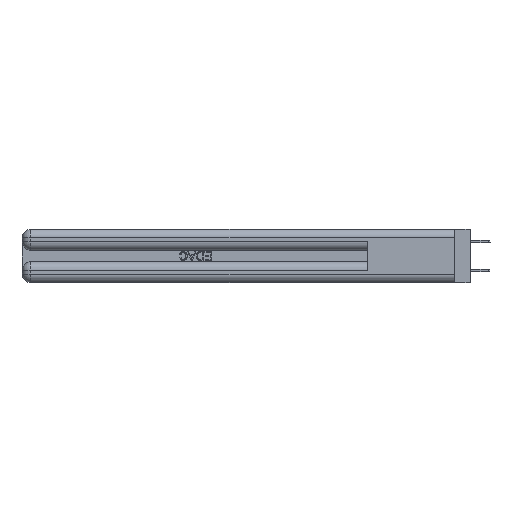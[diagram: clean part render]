
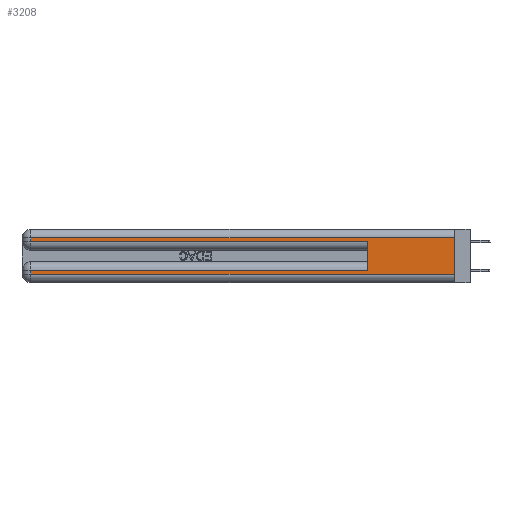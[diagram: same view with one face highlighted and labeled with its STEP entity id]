
A CAD part, left-side view. The second image highlights one B-rep face of the part: STEP entity #3208.
In plain terms, the highlighted planar face has unit normal (-1, 0, 0).
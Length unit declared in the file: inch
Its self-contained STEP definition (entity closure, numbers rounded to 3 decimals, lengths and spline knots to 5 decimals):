
#402 = LINE ( 'NONE', #8190, #17133 ) ;
#724 = ORIENTED_EDGE ( 'NONE', *, *, #35817, .T. ) ;
#920 = LINE ( 'NONE', #37962, #13564 ) ;
#1256 = CARTESIAN_POINT ( 'NONE',  ( 0., 2.94, 0.285 ) ) ;
#3208 = ADVANCED_FACE ( 'NONE', ( #21917 ), #18503, .F. ) ;
#3704 = CARTESIAN_POINT ( 'NONE',  ( 0., 2.94, 0.06 ) ) ;
#3774 = VECTOR ( 'NONE', #37462, 39.37008 ) ;
#5827 = CARTESIAN_POINT ( 'NONE',  ( 0., 0., 0.285 ) ) ;
#7094 = VERTEX_POINT ( 'NONE', #1256 ) ;
#8190 = CARTESIAN_POINT ( 'NONE',  ( 0., 0.6, 0.145 ) ) ;
#8441 = ORIENTED_EDGE ( 'NONE', *, *, #11480, .T. ) ;
#8574 = EDGE_CURVE ( 'NONE', #28456, #36794, #402, .T. ) ;
#8646 = ORIENTED_EDGE ( 'NONE', *, *, #19672, .T. ) ;
#8951 = LINE ( 'NONE', #19665, #41482 ) ;
#8973 = LINE ( 'NONE', #5827, #42919 ) ;
#9868 = ORIENTED_EDGE ( 'NONE', *, *, #24619, .T. ) ;
#10101 = DIRECTION ( 'NONE',  ( 0., 0., -1. ) ) ;
#11480 = EDGE_CURVE ( 'NONE', #7094, #36794, #8973, .T. ) ;
#11812 = CARTESIAN_POINT ( 'NONE',  ( 0., 2.94, 0.31 ) ) ;
#13464 = EDGE_CURVE ( 'NONE', #13974, #33617, #8951, .T. ) ;
#13564 = VECTOR ( 'NONE', #24440, 39.37008 ) ;
#13974 = VERTEX_POINT ( 'NONE', #35438 ) ;
#14116 = CARTESIAN_POINT ( 'NONE',  ( 0., 0., 0.37 ) ) ;
#15988 = VERTEX_POINT ( 'NONE', #47004 ) ;
#17133 = VECTOR ( 'NONE', #18665, 39.37008 ) ;
#18503 = PLANE ( 'NONE',  #19162 ) ;
#18665 = DIRECTION ( 'NONE',  ( 0., 0., 1. ) ) ;
#19162 = AXIS2_PLACEMENT_3D ( 'NONE', #14116, #40468, #36805 ) ;
#19665 = CARTESIAN_POINT ( 'NONE',  ( 0., 2.94, 0.37 ) ) ;
#19672 = EDGE_CURVE ( 'NONE', #43202, #7094, #46413, .T. ) ;
#21067 = ORIENTED_EDGE ( 'NONE', *, *, #26391, .T. ) ;
#21917 = FACE_OUTER_BOUND ( 'NONE', #29914, .T. ) ;
#23807 = DIRECTION ( 'NONE',  ( 0., 0., -1. ) ) ;
#24440 = DIRECTION ( 'NONE',  ( 0., 0., -1. ) ) ;
#24619 = EDGE_CURVE ( 'NONE', #28456, #13974, #47533, .T. ) ;
#24631 = DIRECTION ( 'NONE',  ( 0., 1., 0. ) ) ;
#25647 = ORIENTED_EDGE ( 'NONE', *, *, #8574, .F. ) ;
#26391 = EDGE_CURVE ( 'NONE', #15988, #43202, #32862, .T. ) ;
#27746 = CARTESIAN_POINT ( 'NONE',  ( 0., 0.6, 0.085 ) ) ;
#28388 = CARTESIAN_POINT ( 'NONE',  ( 0., 2.94, 0.37 ) ) ;
#28456 = VERTEX_POINT ( 'NONE', #27746 ) ;
#29881 = CARTESIAN_POINT ( 'NONE',  ( 0., 0., 0.06 ) ) ;
#29914 = EDGE_LOOP ( 'NONE', ( #39439, #21067, #8646, #8441, #25647, #9868, #30607, #724 ) ) ;
#30607 = ORIENTED_EDGE ( 'NONE', *, *, #13464, .T. ) ;
#32862 = LINE ( 'NONE', #47722, #45557 ) ;
#33617 = VERTEX_POINT ( 'NONE', #3704 ) ;
#34326 = DIRECTION ( 'NONE',  ( 0., -1., 0. ) ) ;
#35438 = CARTESIAN_POINT ( 'NONE',  ( 0., 2.94, 0.085 ) ) ;
#35817 = EDGE_CURVE ( 'NONE', #33617, #39457, #44999, .T. ) ;
#36137 = VECTOR ( 'NONE', #24631, 39.37008 ) ;
#36330 = CARTESIAN_POINT ( 'NONE',  ( 0., 0., 0.085 ) ) ;
#36794 = VERTEX_POINT ( 'NONE', #47922 ) ;
#36805 = DIRECTION ( 'NONE',  ( 0., 0., -1. ) ) ;
#37462 = DIRECTION ( 'NONE',  ( 0., -1., 0. ) ) ;
#37962 = CARTESIAN_POINT ( 'NONE',  ( 0., 0., 0.37 ) ) ;
#38259 = CARTESIAN_POINT ( 'NONE',  ( 0., 0., 0.06 ) ) ;
#39439 = ORIENTED_EDGE ( 'NONE', *, *, #44683, .F. ) ;
#39457 = VERTEX_POINT ( 'NONE', #38259 ) ;
#39482 = DIRECTION ( 'NONE',  ( 0., 1., 0. ) ) ;
#40468 = DIRECTION ( 'NONE',  ( 1., 0., 0. ) ) ;
#41482 = VECTOR ( 'NONE', #23807, 39.37008 ) ;
#42919 = VECTOR ( 'NONE', #34326, 39.37008 ) ;
#43202 = VERTEX_POINT ( 'NONE', #11812 ) ;
#44495 = VECTOR ( 'NONE', #10101, 39.37008 ) ;
#44683 = EDGE_CURVE ( 'NONE', #15988, #39457, #920, .T. ) ;
#44999 = LINE ( 'NONE', #29881, #3774 ) ;
#45557 = VECTOR ( 'NONE', #39482, 39.37008 ) ;
#46413 = LINE ( 'NONE', #28388, #44495 ) ;
#47004 = CARTESIAN_POINT ( 'NONE',  ( 0., 0., 0.31 ) ) ;
#47533 = LINE ( 'NONE', #36330, #36137 ) ;
#47722 = CARTESIAN_POINT ( 'NONE',  ( 0., 0., 0.31 ) ) ;
#47922 = CARTESIAN_POINT ( 'NONE',  ( 0., 0.6, 0.285 ) ) ;
